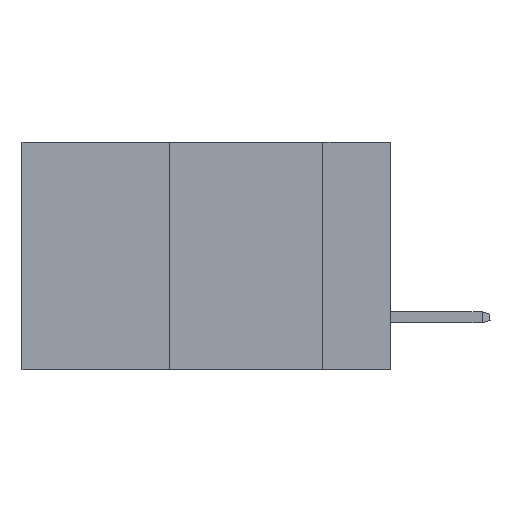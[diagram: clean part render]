
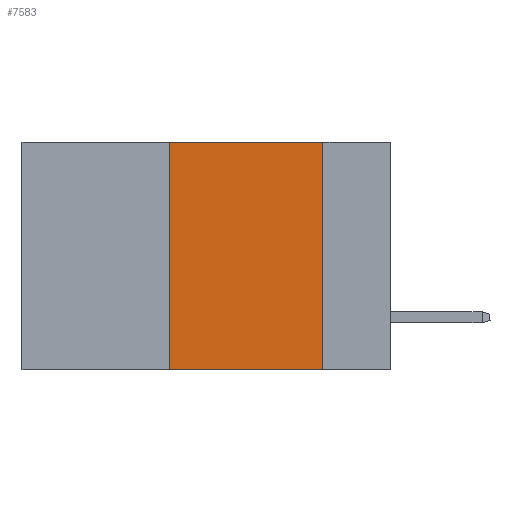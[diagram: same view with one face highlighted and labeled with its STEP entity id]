
A CAD part, left-side view. The second image highlights one B-rep face of the part: STEP entity #7583.
In plain terms, the highlighted planar face has unit normal (-1, 0, 0).
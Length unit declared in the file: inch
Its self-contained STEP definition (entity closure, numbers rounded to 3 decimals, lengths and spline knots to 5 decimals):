
#366 = VERTEX_POINT ( 'NONE', #8940 ) ;
#438 = CARTESIAN_POINT ( 'NONE',  ( 0., 0.6, 0. ) ) ;
#3532 = FACE_OUTER_BOUND ( 'NONE', #4554, .T. ) ;
#4554 = EDGE_LOOP ( 'NONE', ( #10502, #22111, #24730, #15681 ) ) ;
#4574 = CARTESIAN_POINT ( 'NONE',  ( 0., 0.11, -0.37 ) ) ;
#5146 = CARTESIAN_POINT ( 'NONE',  ( 0., 0.36, -0.37 ) ) ;
#5519 = PLANE ( 'NONE',  #29977 ) ;
#5692 = EDGE_CURVE ( 'NONE', #12658, #23413, #15247, .T. ) ;
#5884 = LINE ( 'NONE', #24072, #23086 ) ;
#5937 = VECTOR ( 'NONE', #9909, 39.37008 ) ;
#7583 = ADVANCED_FACE ( 'NONE', ( #3532 ), #5519, .F. ) ;
#8112 = CARTESIAN_POINT ( 'NONE',  ( 0., 0.36, 0. ) ) ;
#8512 = CARTESIAN_POINT ( 'NONE',  ( 0., 0.6, -0.37 ) ) ;
#8940 = CARTESIAN_POINT ( 'NONE',  ( 0., 0.11, 0. ) ) ;
#9132 = DIRECTION ( 'NONE',  ( 0., 0., -1. ) ) ;
#9909 = DIRECTION ( 'NONE',  ( 0., -1., 0. ) ) ;
#10065 = VERTEX_POINT ( 'NONE', #4574 ) ;
#10502 = ORIENTED_EDGE ( 'NONE', *, *, #15073, .F. ) ;
#12658 = VERTEX_POINT ( 'NONE', #5146 ) ;
#12756 = CARTESIAN_POINT ( 'NONE',  ( 0., 0.6, 0. ) ) ;
#13042 = DIRECTION ( 'NONE',  ( 0., -1., 0. ) ) ;
#14388 = EDGE_CURVE ( 'NONE', #12658, #10065, #31767, .T. ) ;
#15073 = EDGE_CURVE ( 'NONE', #366, #10065, #5884, .T. ) ;
#15247 = LINE ( 'NONE', #8112, #26677 ) ;
#15681 = ORIENTED_EDGE ( 'NONE', *, *, #14388, .T. ) ;
#17910 = DIRECTION ( 'NONE',  ( 1., 0., 0. ) ) ;
#19191 = LINE ( 'NONE', #12756, #5937 ) ;
#19195 = VECTOR ( 'NONE', #13042, 39.37008 ) ;
#20910 = DIRECTION ( 'NONE',  ( 0., 0., 1. ) ) ;
#22111 = ORIENTED_EDGE ( 'NONE', *, *, #28819, .F. ) ;
#23086 = VECTOR ( 'NONE', #9132, 39.37008 ) ;
#23413 = VERTEX_POINT ( 'NONE', #23621 ) ;
#23621 = CARTESIAN_POINT ( 'NONE',  ( 0., 0.36, 0. ) ) ;
#24072 = CARTESIAN_POINT ( 'NONE',  ( 0., 0.11, 0. ) ) ;
#24730 = ORIENTED_EDGE ( 'NONE', *, *, #5692, .F. ) ;
#26677 = VECTOR ( 'NONE', #20910, 39.37008 ) ;
#28119 = DIRECTION ( 'NONE',  ( 0., 0., -1. ) ) ;
#28819 = EDGE_CURVE ( 'NONE', #23413, #366, #19191, .T. ) ;
#29977 = AXIS2_PLACEMENT_3D ( 'NONE', #438, #17910, #28119 ) ;
#31767 = LINE ( 'NONE', #8512, #19195 ) ;
